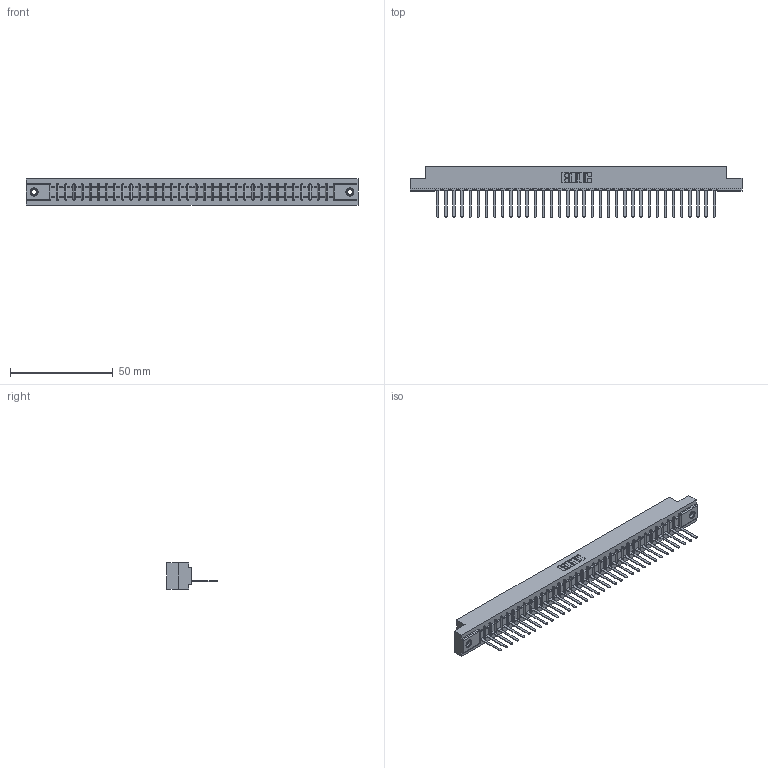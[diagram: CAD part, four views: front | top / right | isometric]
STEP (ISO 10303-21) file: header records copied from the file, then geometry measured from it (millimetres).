
FILE_DESCRIPTION (( 'STEP AP203' ), '1' );
FILE_NAME ('307-035-441-107.STEP', '2020-09-28T23:32:39', ( '' ), ( '' ), 'SwSTEP 2.0', 'SolidWorks 2020', '' );
FILE_SCHEMA (( 'CONFIG_CONTROL_DESIGN' ));
Length unit declared in the file: inch
Products named in the file (4): 307-290-002_541; 307 Part_.156 Dia Mounting Holes; 345-250-001_345-250-005-103; 307-035-441-107
Assembly tree (38 placements, depth 2):
  307-035-441-107
    307 Part_.156 Dia Mounting Holes
    307-290-002_541  x35
    345-250-001_345-250-005-103  x2
Bounding box: 161.7 x 24.59 x 12.7 mm (x, y, z)
Volume: 17336.6 mm3; surface area: 22313.2 mm2
Topology: 38 solids, 38 shells, 2804 faces, 8579 edges, 5614 vertices
Faces by surface type: plane 1677, cylinder 1039, sphere 72, cone 12, torus 4
Entity records: 32771 total; most frequent: CARTESIAN_POINT 5507, ORIENTED_EDGE 5490, DIRECTION 5363, EDGE_CURVE 2745, LINE 2099, VECTOR 2099, VERTEX_POINT 1776, AXIS2_PLACEMENT_3D 1632
